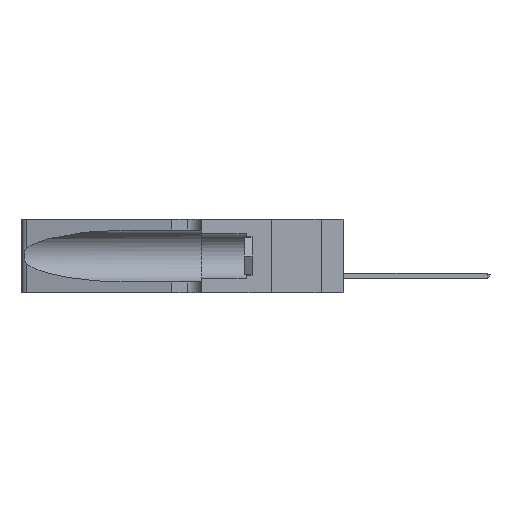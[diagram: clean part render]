
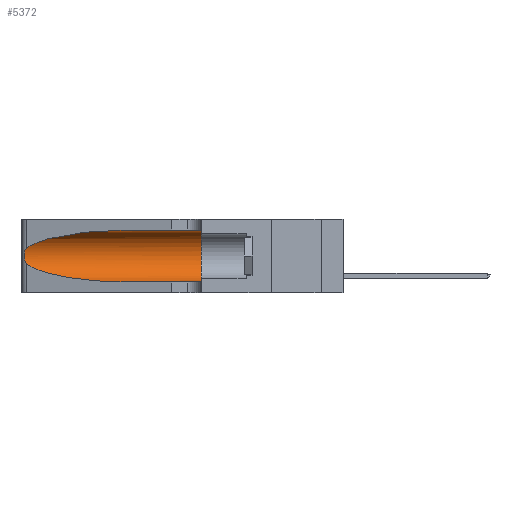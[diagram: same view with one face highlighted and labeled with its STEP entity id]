
A CAD part, left-side view. The second image highlights one B-rep face of the part: STEP entity #5372.
In plain terms, the highlighted cylindrical face has radius 3.308 mm (diameter 6.617 mm), a partial arc.
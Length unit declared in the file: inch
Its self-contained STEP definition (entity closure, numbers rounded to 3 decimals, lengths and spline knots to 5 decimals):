
#537 = DIRECTION ( 'NONE',  ( 0., 1., 0. ) ) ;
#575 = CARTESIAN_POINT ( 'NONE',  ( 0.25639, 1.23184, 0.21858 ) ) ;
#658 = CARTESIAN_POINT ( 'NONE',  ( 0.26017, 1.23833, 0.17102 ) ) ;
#1892 = CARTESIAN_POINT ( 'NONE',  ( 0.1305, 0.72297, 0.31525 ) ) ;
#1985 =( BOUNDED_CURVE ( )  B_SPLINE_CURVE ( 3, ( #1892, #14632, #3768, #3926 ),
 .UNSPECIFIED., .F., .T. ) 
 B_SPLINE_CURVE_WITH_KNOTS ( ( 4, 4 ),
 ( 1.5708, 2.84003 ),
 .UNSPECIFIED. ) 
 CURVE ( )  GEOMETRIC_REPRESENTATION_ITEM ( )  RATIONAL_B_SPLINE_CURVE ( ( 1., 0.87, 0.87, 1. ) ) 
 REPRESENTATION_ITEM ( '' )  );
#2150 = VERTEX_POINT ( 'NONE', #14034 ) ;
#2324 = DIRECTION ( 'NONE',  ( 0., 0., 1. ) ) ;
#2358 = DIRECTION ( 'NONE',  ( 0., -1., 0. ) ) ;
#2521 = CARTESIAN_POINT ( 'NONE',  ( 0.25639, 1.23186, 0.15144 ) ) ;
#2555 = CARTESIAN_POINT ( 'NONE',  ( 0.1305, 0.35, 0.185 ) ) ;
#2872 = CARTESIAN_POINT ( 'NONE',  ( 0.18966, 0.96281, 0.05475 ) ) ;
#3351 = CARTESIAN_POINT ( 'NONE',  ( 0.1305, 0.35, 0.05475 ) ) ;
#3768 = CARTESIAN_POINT ( 'NONE',  ( 0.2373, 1.15595, 0.28018 ) ) ;
#3926 = CARTESIAN_POINT ( 'NONE',  ( 0.25487, 1.22718, 0.22369 ) ) ;
#4046 = EDGE_CURVE ( 'NONE', #12457, #15953, #1985, .T. ) ;
#4060 = CARTESIAN_POINT ( 'NONE',  ( 0.2373, 1.15595, 0.08982 ) ) ;
#4117 = ORIENTED_EDGE ( 'NONE', *, *, #19508, .T. ) ;
#4281 = CARTESIAN_POINT ( 'NONE',  ( 0.25555, 1.22994, 0.2215 ) ) ;
#4529 = CARTESIAN_POINT ( 'NONE',  ( 0.25487, 1.22718, 0.14631 ) ) ;
#5372 = ADVANCED_FACE ( 'NONE', ( #21448 ), #8911, .F. ) ;
#5816 = CARTESIAN_POINT ( 'NONE',  ( 0.25856, 1.23593, 0.16098 ) ) ;
#6003 = CARTESIAN_POINT ( 'NONE',  ( 0.1305, 1.61858, 0.185 ) ) ;
#6890 = VERTEX_POINT ( 'NONE', #10663 ) ;
#7246 = ORIENTED_EDGE ( 'NONE', *, *, #12777, .F. ) ;
#7536 = CARTESIAN_POINT ( 'NONE',  ( 0.1305, 1.61858, 0.31525 ) ) ;
#7579 = CARTESIAN_POINT ( 'NONE',  ( 0.25487, 1.22718, 0.14631 ) ) ;
#7619 = CARTESIAN_POINT ( 'NONE',  ( 0.1305, 0.72297, 0.31525 ) ) ;
#7620 = ORIENTED_EDGE ( 'NONE', *, *, #4046, .T. ) ;
#7626 = CARTESIAN_POINT ( 'NONE',  ( 0.25789, 1.23486, 0.15765 ) ) ;
#7806 = CARTESIAN_POINT ( 'NONE',  ( 0.1305, 1.61858, 0.05475 ) ) ;
#8193 = CARTESIAN_POINT ( 'NONE',  ( 0.1305, 0.72297, 0.05475 ) ) ;
#8636 = EDGE_CURVE ( 'NONE', #2150, #10931, #9719, .T. ) ;
#8806 = EDGE_LOOP ( 'NONE', ( #7620, #4117, #19127, #14836, #9439, #7246 ) ) ;
#8911 = CYLINDRICAL_SURFACE ( 'NONE', #16235, 0.13025 ) ;
#8965 = CIRCLE ( 'NONE', #21517, 0.13025 ) ;
#9161 = VERTEX_POINT ( 'NONE', #4529 ) ;
#9292 = EDGE_CURVE ( 'NONE', #9161, #2150, #10349, .T. ) ;
#9439 = ORIENTED_EDGE ( 'NONE', *, *, #13093, .F. ) ;
#9445 = CARTESIAN_POINT ( 'NONE',  ( 0.26018, 1.23835, 0.19895 ) ) ;
#9719 = LINE ( 'NONE', #7806, #19218 ) ;
#10349 =( BOUNDED_CURVE ( )  B_SPLINE_CURVE ( 3, ( #7579, #4060, #2872, #8193 ),
 .UNSPECIFIED., .F., .T. ) 
 B_SPLINE_CURVE_WITH_KNOTS ( ( 4, 4 ),
 ( 3.44316, 4.71239 ),
 .UNSPECIFIED. ) 
 CURVE ( )  GEOMETRIC_REPRESENTATION_ITEM ( )  RATIONAL_B_SPLINE_CURVE ( ( 1., 0.87, 0.87, 1. ) ) 
 REPRESENTATION_ITEM ( '' )  );
#10663 = CARTESIAN_POINT ( 'NONE',  ( 0.1305, 0.35, 0.31525 ) ) ;
#10931 = VERTEX_POINT ( 'NONE', #3351 ) ;
#12457 = VERTEX_POINT ( 'NONE', #7619 ) ;
#12777 = EDGE_CURVE ( 'NONE', #12457, #6890, #17366, .T. ) ;
#12927 = CARTESIAN_POINT ( 'NONE',  ( 0.25854, 1.2359, 0.20912 ) ) ;
#13093 = EDGE_CURVE ( 'NONE', #6890, #10931, #8965, .T. ) ;
#13098 = CARTESIAN_POINT ( 'NONE',  ( 0.25787, 1.23484, 0.2124 ) ) ;
#13203 = DIRECTION ( 'NONE',  ( 0., -1., 0. ) ) ;
#14034 = CARTESIAN_POINT ( 'NONE',  ( 0.1305, 0.72297, 0.05475 ) ) ;
#14632 = CARTESIAN_POINT ( 'NONE',  ( 0.18966, 0.96281, 0.31525 ) ) ;
#14836 = ORIENTED_EDGE ( 'NONE', *, *, #8636, .T. ) ;
#14922 = CARTESIAN_POINT ( 'NONE',  ( 0.26075, 1.23896, 0.178 ) ) ;
#15953 = VERTEX_POINT ( 'NONE', #19536 ) ;
#16235 = AXIS2_PLACEMENT_3D ( 'NONE', #6003, #13203, #18527 ) ;
#16777 = CARTESIAN_POINT ( 'NONE',  ( 0.25555, 1.22993, 0.14849 ) ) ;
#17366 = LINE ( 'NONE', #7536, #20975 ) ;
#18527 = DIRECTION ( 'NONE',  ( 0., 0., -1. ) ) ;
#18578 = CARTESIAN_POINT ( 'NONE',  ( 0.25487, 1.22718, 0.14631 ) ) ;
#18660 = CARTESIAN_POINT ( 'NONE',  ( 0.26075, 1.23896, 0.19203 ) ) ;
#19127 = ORIENTED_EDGE ( 'NONE', *, *, #9292, .T. ) ;
#19218 = VECTOR ( 'NONE', #2358, 39.37008 ) ;
#19508 = EDGE_CURVE ( 'NONE', #15953, #9161, #20054, .T. ) ;
#19536 = CARTESIAN_POINT ( 'NONE',  ( 0.25487, 1.22718, 0.22369 ) ) ;
#20054 = B_SPLINE_CURVE_WITH_KNOTS ( 'NONE', 3,
 ( #20202, #4281, #575, #13098, #12927, #9445, #18660, #14922, #658, #5816, #7626, #2521, #16777, #18578 ),
 .UNSPECIFIED., .F., .F.,
 ( 4, 2, 2, 2, 2, 2, 4 ),
 ( 0., 0.00027, 0.00053, 0.00107, 0.0016, 0.00187, 0.00214 ),
 .UNSPECIFIED. ) ;
#20116 = DIRECTION ( 'NONE',  ( 0., -1., 0. ) ) ;
#20202 = CARTESIAN_POINT ( 'NONE',  ( 0.25487, 1.22718, 0.22369 ) ) ;
#20975 = VECTOR ( 'NONE', #20116, 39.37008 ) ;
#21448 = FACE_OUTER_BOUND ( 'NONE', #8806, .T. ) ;
#21517 = AXIS2_PLACEMENT_3D ( 'NONE', #2555, #537, #2324 ) ;
